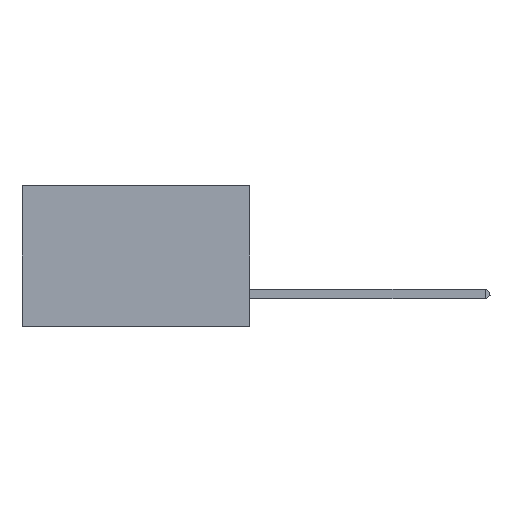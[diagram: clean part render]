
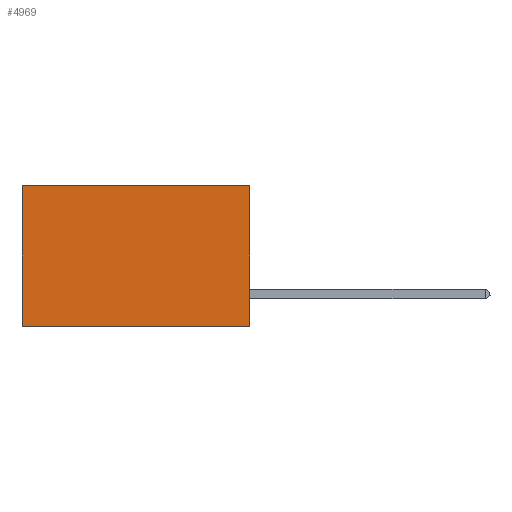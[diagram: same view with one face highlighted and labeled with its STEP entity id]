
A CAD part, left-side view. The second image highlights one B-rep face of the part: STEP entity #4969.
In plain terms, the highlighted planar face has unit normal (-1, 0, 0).
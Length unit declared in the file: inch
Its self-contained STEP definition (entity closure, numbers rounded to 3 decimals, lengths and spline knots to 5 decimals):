
#521 = VECTOR ( 'NONE', #20975, 39.37008 ) ;
#537 = DIRECTION ( 'NONE',  ( 0., 0., -1. ) ) ;
#2209 = CARTESIAN_POINT ( 'NONE',  ( 0.2875, 0., 0. ) ) ;
#4969 = ADVANCED_FACE ( 'NONE', ( #24734 ), #7631, .F. ) ;
#4977 = CARTESIAN_POINT ( 'NONE',  ( 0.2875, 0.6, -0.37 ) ) ;
#7631 = PLANE ( 'NONE',  #10021 ) ;
#7863 = LINE ( 'NONE', #2209, #521 ) ;
#10021 = AXIS2_PLACEMENT_3D ( 'NONE', #40071, #25875, #43724 ) ;
#12076 = CARTESIAN_POINT ( 'NONE',  ( 0.2875, 0., 0. ) ) ;
#12091 = VECTOR ( 'NONE', #12637, 39.37008 ) ;
#12171 = CARTESIAN_POINT ( 'NONE',  ( 0.2875, 0.6, 0. ) ) ;
#12453 = EDGE_CURVE ( 'NONE', #23311, #21549, #30764, .T. ) ;
#12637 = DIRECTION ( 'NONE',  ( 0., 1., 0. ) ) ;
#14470 = VERTEX_POINT ( 'NONE', #4977 ) ;
#14861 = CARTESIAN_POINT ( 'NONE',  ( 0.2875, 0.6, 0. ) ) ;
#19903 = ORIENTED_EDGE ( 'NONE', *, *, #12453, .T. ) ;
#20975 = DIRECTION ( 'NONE',  ( 0., 0., -1. ) ) ;
#21549 = VERTEX_POINT ( 'NONE', #12171 ) ;
#21737 = EDGE_CURVE ( 'NONE', #42412, #14470, #35907, .T. ) ;
#23090 = CARTESIAN_POINT ( 'NONE',  ( 0.2875, 0., -0.37 ) ) ;
#23311 = VERTEX_POINT ( 'NONE', #12076 ) ;
#23435 = EDGE_LOOP ( 'NONE', ( #38737, #37062, #25818, #19903 ) ) ;
#23878 = CARTESIAN_POINT ( 'NONE',  ( 0.2875, 0., 0. ) ) ;
#24734 = FACE_OUTER_BOUND ( 'NONE', #23435, .T. ) ;
#25818 = ORIENTED_EDGE ( 'NONE', *, *, #45772, .F. ) ;
#25875 = DIRECTION ( 'NONE',  ( 1., 0., 0. ) ) ;
#29623 = VECTOR ( 'NONE', #45464, 39.37008 ) ;
#29665 = LINE ( 'NONE', #14861, #38188 ) ;
#30764 = LINE ( 'NONE', #23878, #29623 ) ;
#35907 = LINE ( 'NONE', #45025, #12091 ) ;
#37062 = ORIENTED_EDGE ( 'NONE', *, *, #21737, .F. ) ;
#38188 = VECTOR ( 'NONE', #537, 39.37008 ) ;
#38737 = ORIENTED_EDGE ( 'NONE', *, *, #43236, .T. ) ;
#40071 = CARTESIAN_POINT ( 'NONE',  ( 0.2875, 0., 0. ) ) ;
#42412 = VERTEX_POINT ( 'NONE', #23090 ) ;
#43236 = EDGE_CURVE ( 'NONE', #21549, #14470, #29665, .T. ) ;
#43724 = DIRECTION ( 'NONE',  ( 0., 0., -1. ) ) ;
#45025 = CARTESIAN_POINT ( 'NONE',  ( 0.2875, 0., -0.37 ) ) ;
#45464 = DIRECTION ( 'NONE',  ( 0., 1., 0. ) ) ;
#45772 = EDGE_CURVE ( 'NONE', #23311, #42412, #7863, .T. ) ;
